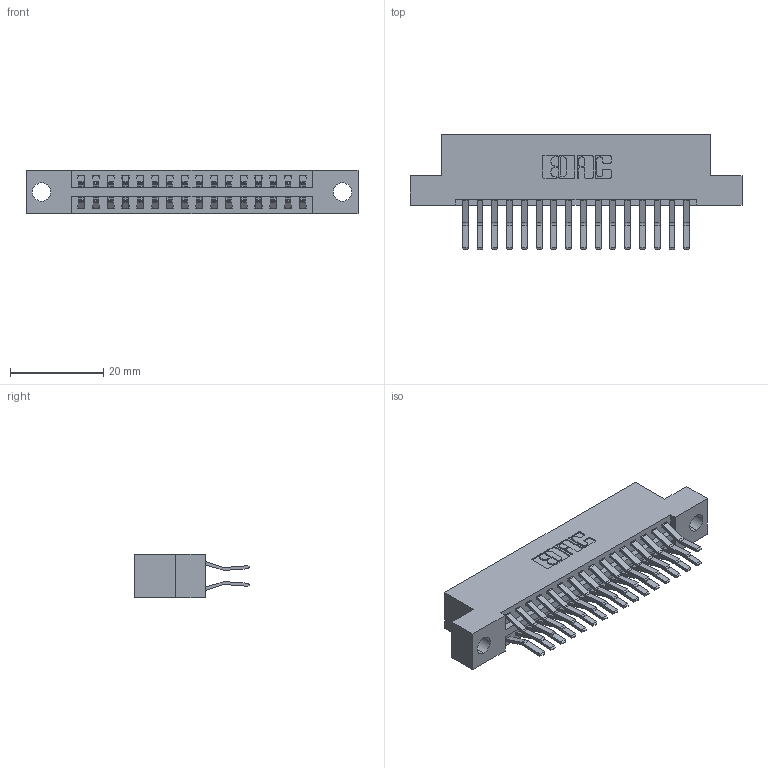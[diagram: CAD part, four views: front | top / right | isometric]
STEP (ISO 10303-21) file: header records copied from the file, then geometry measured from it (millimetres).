
FILE_DESCRIPTION (( 'STEP AP203' ), '1' );
FILE_NAME ('346-032-560-204.STEP', '2022-05-19T18:50:12', ( '' ), ( '' ), 'SwSTEP 2.0', 'SolidWorks 2020', '' );
FILE_SCHEMA (( 'CONFIG_CONTROL_DESIGN' ));
Length unit declared in the file: inch
Products named in the file (3): 346 Part_Flush Mounting Lugs - 0.156 Dia-TH; 346-032-560-204; 345-292-001_560 Tail
Assembly tree (33 placements, depth 2):
  346-032-560-204
    346 Part_Flush Mounting Lugs - 0.156 Dia-TH
    345-292-001_560 Tail  x32
Bounding box: 71.37 x 24.78 x 9.4 mm (x, y, z)
Volume: 6861.7 mm3; surface area: 9430.7 mm2
Topology: 33 solids, 33 shells, 1864 faces, 5517 edges, 3634 vertices
Faces by surface type: plane 1210, cylinder 654
Entity records: 14449 total; most frequent: CARTESIAN_POINT 2422, ORIENTED_EDGE 2354, DIRECTION 2189, EDGE_CURVE 1177, VECTOR 977, LINE 977, VERTEX_POINT 782, AXIS2_PLACEMENT_3D 606
